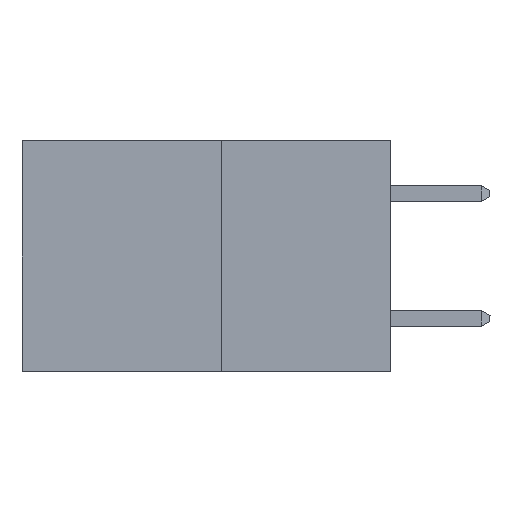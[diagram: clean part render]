
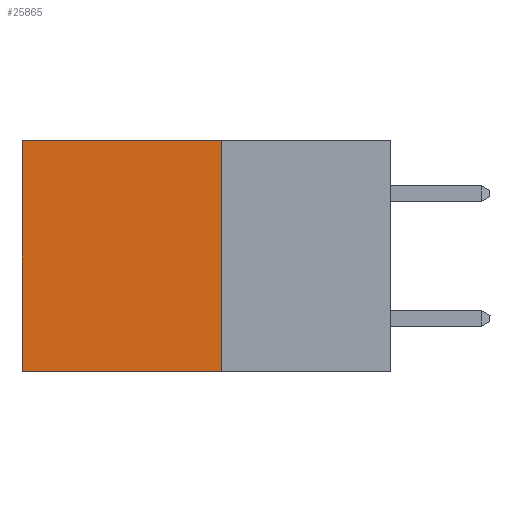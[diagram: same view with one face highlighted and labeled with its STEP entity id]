
A CAD part, left-side view. The second image highlights one B-rep face of the part: STEP entity #25865.
In plain terms, the highlighted planar face has unit normal (-1, 0, 0).
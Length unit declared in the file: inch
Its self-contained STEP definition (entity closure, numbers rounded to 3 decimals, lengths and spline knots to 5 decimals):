
#291 = CARTESIAN_POINT ( 'NONE',  ( 0.277, 0.27, -0.37 ) ) ;
#317 = VECTOR ( 'NONE', #11886, 39.37008 ) ;
#1148 = LINE ( 'NONE', #16871, #14026 ) ;
#1867 = DIRECTION ( 'NONE',  ( 0., 0., -1. ) ) ;
#2902 = DIRECTION ( 'NONE',  ( 0., 0., -1. ) ) ;
#5633 = ORIENTED_EDGE ( 'NONE', *, *, #23701, .T. ) ;
#6570 = AXIS2_PLACEMENT_3D ( 'NONE', #291, #18307, #2902 ) ;
#6653 = VECTOR ( 'NONE', #29258, 39.37008 ) ;
#6871 = CARTESIAN_POINT ( 'NONE',  ( 0.277, 0.59, 0. ) ) ;
#9281 = CARTESIAN_POINT ( 'NONE',  ( 0.277, 0.27, -0.37 ) ) ;
#9497 = CARTESIAN_POINT ( 'NONE',  ( 0.277, 0.59, -0.37 ) ) ;
#10750 = VERTEX_POINT ( 'NONE', #12869 ) ;
#11269 = CARTESIAN_POINT ( 'NONE',  ( 0.277, 0.27, -0.37 ) ) ;
#11886 = DIRECTION ( 'NONE',  ( 0., 0., -1. ) ) ;
#12130 = VERTEX_POINT ( 'NONE', #20583 ) ;
#12869 = CARTESIAN_POINT ( 'NONE',  ( 0.277, 0.27, -0.37 ) ) ;
#14026 = VECTOR ( 'NONE', #29645, 39.37008 ) ;
#14377 = VECTOR ( 'NONE', #1867, 39.37008 ) ;
#16294 = FACE_OUTER_BOUND ( 'NONE', #23969, .T. ) ;
#16871 = CARTESIAN_POINT ( 'NONE',  ( 0.277, 0.27, 0. ) ) ;
#18307 = DIRECTION ( 'NONE',  ( 1., 0., 0. ) ) ;
#20386 = LINE ( 'NONE', #11269, #6653 ) ;
#20583 = CARTESIAN_POINT ( 'NONE',  ( 0.277, 0.27, 0. ) ) ;
#23701 = EDGE_CURVE ( 'NONE', #12130, #29165, #1148, .T. ) ;
#23741 = EDGE_CURVE ( 'NONE', #12130, #10750, #26903, .T. ) ;
#23944 = ORIENTED_EDGE ( 'NONE', *, *, #24435, .T. ) ;
#23969 = EDGE_LOOP ( 'NONE', ( #23944, #30223, #25969, #5633 ) ) ;
#24435 = EDGE_CURVE ( 'NONE', #29165, #25720, #28044, .T. ) ;
#24876 = EDGE_CURVE ( 'NONE', #10750, #25720, #20386, .T. ) ;
#25720 = VERTEX_POINT ( 'NONE', #9497 ) ;
#25865 = ADVANCED_FACE ( 'NONE', ( #16294 ), #25963, .F. ) ;
#25963 = PLANE ( 'NONE',  #6570 ) ;
#25969 = ORIENTED_EDGE ( 'NONE', *, *, #23741, .F. ) ;
#26903 = LINE ( 'NONE', #9281, #317 ) ;
#28044 = LINE ( 'NONE', #32615, #14377 ) ;
#29165 = VERTEX_POINT ( 'NONE', #6871 ) ;
#29258 = DIRECTION ( 'NONE',  ( 0., 1., 0. ) ) ;
#29645 = DIRECTION ( 'NONE',  ( 0., 1., 0. ) ) ;
#30223 = ORIENTED_EDGE ( 'NONE', *, *, #24876, .F. ) ;
#32615 = CARTESIAN_POINT ( 'NONE',  ( 0.277, 0.59, -0.37 ) ) ;
